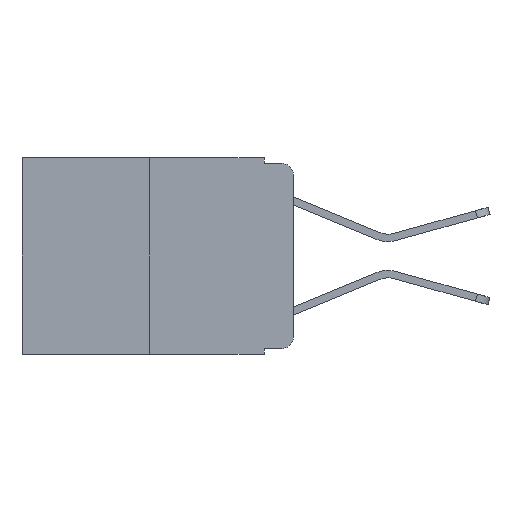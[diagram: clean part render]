
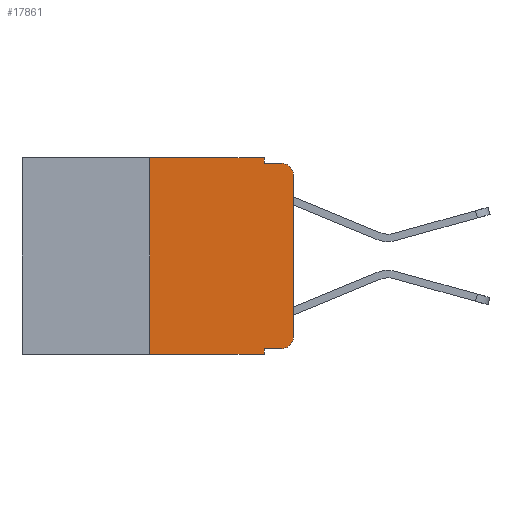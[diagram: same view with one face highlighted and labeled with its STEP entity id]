
A CAD part, left-side view. The second image highlights one B-rep face of the part: STEP entity #17861.
In plain terms, the highlighted planar face has unit normal (-1, 0, 0).
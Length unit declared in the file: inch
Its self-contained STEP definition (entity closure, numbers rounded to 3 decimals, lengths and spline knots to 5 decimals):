
#16 = EDGE_CURVE ( 'NONE', #10269, #14346, #17160, .T. ) ;
#937 = ORIENTED_EDGE ( 'NONE', *, *, #14867, .T. ) ;
#1571 = CARTESIAN_POINT ( 'NONE',  ( 0., 0.051, -0.01 ) ) ;
#1794 = CARTESIAN_POINT ( 'NONE',  ( 0., 0.473, 0. ) ) ;
#1973 = ORIENTED_EDGE ( 'NONE', *, *, #5876, .F. ) ;
#2406 = LINE ( 'NONE', #2868, #10293 ) ;
#2535 = VECTOR ( 'NONE', #8984, 39.37008 ) ;
#2868 = CARTESIAN_POINT ( 'NONE',  ( 0., 0.051, -0.333 ) ) ;
#3438 = DIRECTION ( 'NONE',  ( 0., 0., -1. ) ) ;
#3951 = CARTESIAN_POINT ( 'NONE',  ( 0., 0.051, -0.333 ) ) ;
#4203 = VERTEX_POINT ( 'NONE', #19084 ) ;
#4259 = CARTESIAN_POINT ( 'NONE',  ( 0., 0.473, 0. ) ) ;
#4756 = AXIS2_PLACEMENT_3D ( 'NONE', #17483, #8310, #19021 ) ;
#5103 = VECTOR ( 'NONE', #9686, 39.37008 ) ;
#5259 = ORIENTED_EDGE ( 'NONE', *, *, #10695, .T. ) ;
#5355 = VECTOR ( 'NONE', #13663, 39.37008 ) ;
#5520 = AXIS2_PLACEMENT_3D ( 'NONE', #1794, #12816, #3438 ) ;
#5760 = CARTESIAN_POINT ( 'NONE',  ( 0., 0.051, 0. ) ) ;
#5876 = EDGE_CURVE ( 'NONE', #10269, #13474, #17616, .T. ) ;
#6233 = ORIENTED_EDGE ( 'NONE', *, *, #16, .T. ) ;
#6711 = ORIENTED_EDGE ( 'NONE', *, *, #12512, .F. ) ;
#6759 = LINE ( 'NONE', #4259, #2535 ) ;
#6825 = VERTEX_POINT ( 'NONE', #12957 ) ;
#7950 = EDGE_CURVE ( 'NONE', #16868, #8810, #15888, .T. ) ;
#8129 = VERTEX_POINT ( 'NONE', #8647 ) ;
#8310 = DIRECTION ( 'NONE',  ( -1., 0., 0. ) ) ;
#8355 = CIRCLE ( 'NONE', #10876, 0.02 ) ;
#8647 = CARTESIAN_POINT ( 'NONE',  ( 0., 0., -0.313 ) ) ;
#8742 = CARTESIAN_POINT ( 'NONE',  ( 0., 0.25, -0.343 ) ) ;
#8810 = VERTEX_POINT ( 'NONE', #1571 ) ;
#8984 = DIRECTION ( 'NONE',  ( 0., -1., 0. ) ) ;
#9379 = EDGE_CURVE ( 'NONE', #13523, #8129, #8355, .T. ) ;
#9440 = CARTESIAN_POINT ( 'NONE',  ( 0., 0.02, -0.313 ) ) ;
#9686 = DIRECTION ( 'NONE',  ( 0., 0., 1. ) ) ;
#9702 = EDGE_LOOP ( 'NONE', ( #937, #5259, #13508, #17526, #13994, #1973, #6233, #6711, #10851, #14976 ) ) ;
#9954 = CARTESIAN_POINT ( 'NONE',  ( 0., 0.051, 0. ) ) ;
#10269 = VERTEX_POINT ( 'NONE', #8742 ) ;
#10293 = VECTOR ( 'NONE', #13810, 39.37008 ) ;
#10362 = VECTOR ( 'NONE', #15608, 39.37008 ) ;
#10426 = EDGE_CURVE ( 'NONE', #17437, #13523, #2406, .T. ) ;
#10695 = EDGE_CURVE ( 'NONE', #4203, #6825, #13657, .T. ) ;
#10851 = ORIENTED_EDGE ( 'NONE', *, *, #10426, .T. ) ;
#10876 = AXIS2_PLACEMENT_3D ( 'NONE', #9440, #20093, #11011 ) ;
#11011 = DIRECTION ( 'NONE',  ( 0., 0., -1. ) ) ;
#11256 = PLANE ( 'NONE',  #5520 ) ;
#12128 = EDGE_CURVE ( 'NONE', #8810, #6825, #15758, .T. ) ;
#12133 = CARTESIAN_POINT ( 'NONE',  ( 0., 0.25, 0. ) ) ;
#12512 = EDGE_CURVE ( 'NONE', #17437, #14346, #12627, .T. ) ;
#12627 = LINE ( 'NONE', #5760, #20172 ) ;
#12777 = FACE_OUTER_BOUND ( 'NONE', #9702, .T. ) ;
#12816 = DIRECTION ( 'NONE',  ( 1., 0., 0. ) ) ;
#12957 = CARTESIAN_POINT ( 'NONE',  ( 0., 0.02, -0.01 ) ) ;
#13050 = CARTESIAN_POINT ( 'NONE',  ( 0., 0.25, 0. ) ) ;
#13144 = VECTOR ( 'NONE', #15772, 39.37008 ) ;
#13358 = LINE ( 'NONE', #18844, #5103 ) ;
#13474 = VERTEX_POINT ( 'NONE', #13050 ) ;
#13508 = ORIENTED_EDGE ( 'NONE', *, *, #12128, .F. ) ;
#13523 = VERTEX_POINT ( 'NONE', #19216 ) ;
#13547 = DIRECTION ( 'NONE',  ( 0., 0., -1. ) ) ;
#13657 = CIRCLE ( 'NONE', #4756, 0.02 ) ;
#13663 = DIRECTION ( 'NONE',  ( 0., 0., 1. ) ) ;
#13810 = DIRECTION ( 'NONE',  ( 0., -1., 0. ) ) ;
#13994 = ORIENTED_EDGE ( 'NONE', *, *, #15834, .F. ) ;
#14058 = CARTESIAN_POINT ( 'NONE',  ( 0., 0.051, 0. ) ) ;
#14175 = CARTESIAN_POINT ( 'NONE',  ( 0., 0.051, -0.01 ) ) ;
#14346 = VERTEX_POINT ( 'NONE', #15898 ) ;
#14355 = CARTESIAN_POINT ( 'NONE',  ( 0., 0.473, -0.343 ) ) ;
#14867 = EDGE_CURVE ( 'NONE', #8129, #4203, #13358, .T. ) ;
#14976 = ORIENTED_EDGE ( 'NONE', *, *, #9379, .T. ) ;
#15299 = VECTOR ( 'NONE', #15710, 39.37008 ) ;
#15608 = DIRECTION ( 'NONE',  ( 0., 0., -1. ) ) ;
#15710 = DIRECTION ( 'NONE',  ( 0., -1., 0. ) ) ;
#15758 = LINE ( 'NONE', #14175, #15299 ) ;
#15772 = DIRECTION ( 'NONE',  ( 0., -1., 0. ) ) ;
#15834 = EDGE_CURVE ( 'NONE', #13474, #16868, #6759, .T. ) ;
#15888 = LINE ( 'NONE', #14058, #10362 ) ;
#15898 = CARTESIAN_POINT ( 'NONE',  ( 0., 0.051, -0.343 ) ) ;
#16868 = VERTEX_POINT ( 'NONE', #9954 ) ;
#17160 = LINE ( 'NONE', #14355, #13144 ) ;
#17437 = VERTEX_POINT ( 'NONE', #3951 ) ;
#17483 = CARTESIAN_POINT ( 'NONE',  ( 0., 0.02, -0.03 ) ) ;
#17526 = ORIENTED_EDGE ( 'NONE', *, *, #7950, .F. ) ;
#17616 = LINE ( 'NONE', #12133, #5355 ) ;
#17861 = ADVANCED_FACE ( 'NONE', ( #12777 ), #11256, .F. ) ;
#18844 = CARTESIAN_POINT ( 'NONE',  ( 0., 0., 0. ) ) ;
#19021 = DIRECTION ( 'NONE',  ( 0., 0., -1. ) ) ;
#19084 = CARTESIAN_POINT ( 'NONE',  ( 0., 0., -0.03 ) ) ;
#19216 = CARTESIAN_POINT ( 'NONE',  ( 0., 0.02, -0.333 ) ) ;
#20093 = DIRECTION ( 'NONE',  ( -1., 0., 0. ) ) ;
#20172 = VECTOR ( 'NONE', #13547, 39.37008 ) ;
